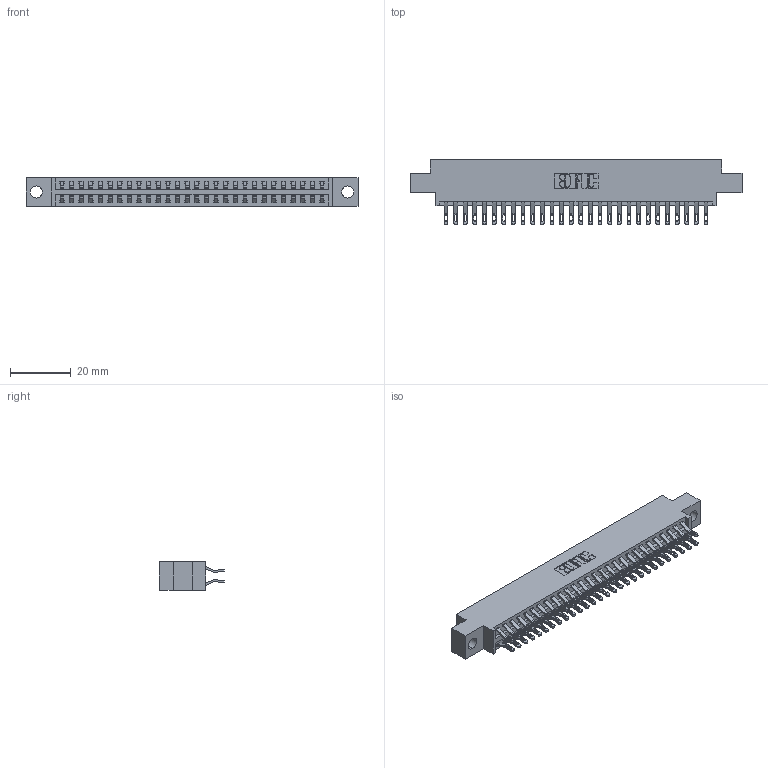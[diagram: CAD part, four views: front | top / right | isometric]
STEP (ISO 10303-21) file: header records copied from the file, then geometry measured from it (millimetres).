
FILE_DESCRIPTION (( 'STEP AP203' ), '1' );
FILE_NAME ('396-056-555-804.STEP', '2019-11-02T08:24:05', ( '' ), ( '' ), 'SwSTEP 2.0', 'SolidWorks 2016', '' );
FILE_SCHEMA (( 'CONFIG_CONTROL_DESIGN' ));
Length unit declared in the file: inch
Products named in the file (3): 345-292-001_555 Tail; 396-056-555-804; 346 Part_0.170 Offset - 0.156 Dia-TH
Assembly tree (57 placements, depth 2):
  396-056-555-804
    346 Part_0.170 Offset - 0.156 Dia-TH
    345-292-001_555 Tail  x56
Bounding box: 109.47 x 21.46 x 9.4 mm (x, y, z)
Volume: 10486.3 mm3; surface area: 14766.1 mm2
Topology: 57 solids, 57 shells, 3374 faces, 10589 edges, 7058 vertices
Faces by surface type: plane 1928, cylinder 1446
Entity records: 20619 total; most frequent: CARTESIAN_POINT 3454, ORIENTED_EDGE 3358, DIRECTION 3063, EDGE_CURVE 1679, VECTOR 1415, LINE 1415, VERTEX_POINT 1118, AXIS2_PLACEMENT_3D 824
